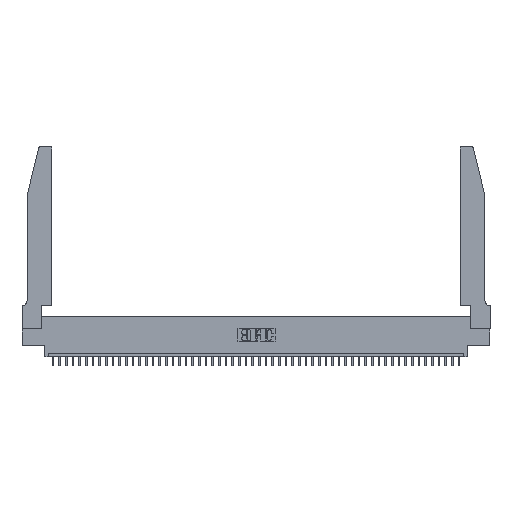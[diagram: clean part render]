
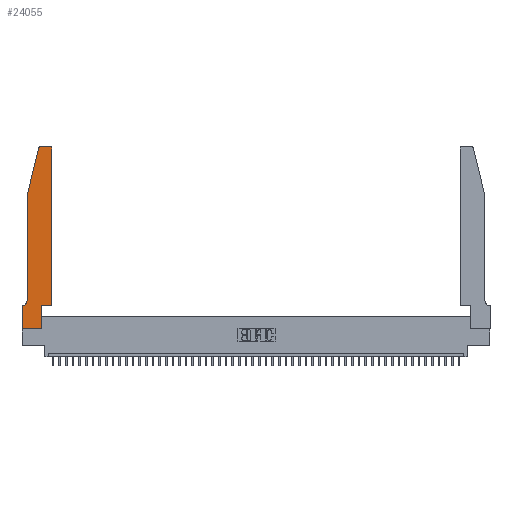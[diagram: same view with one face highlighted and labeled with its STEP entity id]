
A CAD part, top view. The second image highlights one B-rep face of the part: STEP entity #24055.
In plain terms, the highlighted planar face has unit normal (0, 0, 1).
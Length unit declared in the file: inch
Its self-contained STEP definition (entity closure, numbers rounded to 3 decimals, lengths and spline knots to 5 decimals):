
#559 = VECTOR ( 'NONE', #22969, 39.37008 ) ;
#1103 = LINE ( 'NONE', #23574, #22362 ) ;
#1357 = ORIENTED_EDGE ( 'NONE', *, *, #5069, .T. ) ;
#1638 = CARTESIAN_POINT ( 'NONE',  ( 0.0755, 2., 0.37 ) ) ;
#2776 = VERTEX_POINT ( 'NONE', #11115 ) ;
#2872 = DIRECTION ( 'NONE',  ( -1., 0., 0. ) ) ;
#3125 = DIRECTION ( 'NONE',  ( 1., 0., 0. ) ) ;
#4115 = ORIENTED_EDGE ( 'NONE', *, *, #41771, .T. ) ;
#4486 = VECTOR ( 'NONE', #7518, 39.37008 ) ;
#4956 = EDGE_CURVE ( 'NONE', #36904, #31298, #45516, .T. ) ;
#5069 = EDGE_CURVE ( 'NONE', #30565, #15006, #5360, .T. ) ;
#5360 = LINE ( 'NONE', #42380, #559 ) ;
#6706 = DIRECTION ( 'NONE',  ( 1., 0., 0. ) ) ;
#7518 = DIRECTION ( 'NONE',  ( 0., 1., 0. ) ) ;
#7743 = LINE ( 'NONE', #1638, #20049 ) ;
#8378 = CARTESIAN_POINT ( 'NONE',  ( 0.25487, 2.72718, 0.37 ) ) ;
#9094 = LINE ( 'NONE', #27854, #23167 ) ;
#9444 = ORIENTED_EDGE ( 'NONE', *, *, #26801, .T. ) ;
#9681 = AXIS2_PLACEMENT_3D ( 'NONE', #30331, #41600, #33811 ) ;
#9833 = CARTESIAN_POINT ( 'NONE',  ( 0.2865, 0.35, 0.37 ) ) ;
#9986 = ORIENTED_EDGE ( 'NONE', *, *, #24426, .T. ) ;
#10531 = VERTEX_POINT ( 'NONE', #17291 ) ;
#11115 = CARTESIAN_POINT ( 'NONE',  ( 0., 0.35, 0.37 ) ) ;
#11484 = FACE_OUTER_BOUND ( 'NONE', #29767, .T. ) ;
#11718 = CARTESIAN_POINT ( 'NONE',  ( 0.2865, 0., 0.37 ) ) ;
#12061 = DIRECTION ( 'NONE',  ( 0., 1., 0. ) ) ;
#12645 = CARTESIAN_POINT ( 'NONE',  ( 0.0055, 0.35, 0.37 ) ) ;
#12765 = LINE ( 'NONE', #9833, #4486 ) ;
#13331 = CARTESIAN_POINT ( 'NONE',  ( 0.4205, 2.75, 0.37 ) ) ;
#13377 = DIRECTION ( 'NONE',  ( -1., 0., 0. ) ) ;
#14052 = CARTESIAN_POINT ( 'NONE',  ( 0.4205, 2.72, 0.37 ) ) ;
#14626 = AXIS2_PLACEMENT_3D ( 'NONE', #33946, #37298, #3125 ) ;
#15006 = VERTEX_POINT ( 'NONE', #39489 ) ;
#15612 = VECTOR ( 'NONE', #29946, 39.37008 ) ;
#15670 = ORIENTED_EDGE ( 'NONE', *, *, #39494, .T. ) ;
#16817 = AXIS2_PLACEMENT_3D ( 'NONE', #14052, #17802, #6706 ) ;
#17291 = CARTESIAN_POINT ( 'NONE',  ( 0.0755, 0.42, 0.37 ) ) ;
#17571 = EDGE_CURVE ( 'NONE', #15006, #10531, #7743, .T. ) ;
#17802 = DIRECTION ( 'NONE',  ( 0., 0., 1. ) ) ;
#18466 = VERTEX_POINT ( 'NONE', #43878 ) ;
#19421 = VERTEX_POINT ( 'NONE', #13331 ) ;
#20049 = VECTOR ( 'NONE', #35821, 39.37008 ) ;
#20183 = VECTOR ( 'NONE', #25851, 39.37008 ) ;
#20469 = EDGE_CURVE ( 'NONE', #18466, #44618, #1103, .T. ) ;
#21346 = LINE ( 'NONE', #32237, #39133 ) ;
#22362 = VECTOR ( 'NONE', #12061, 39.37008 ) ;
#22926 = VERTEX_POINT ( 'NONE', #47228 ) ;
#22969 = DIRECTION ( 'NONE',  ( -0.239, -0.971, 0. ) ) ;
#23167 = VECTOR ( 'NONE', #41052, 39.37008 ) ;
#23405 = CARTESIAN_POINT ( 'NONE',  ( 0.0055, 0.42, 0.37 ) ) ;
#23574 = CARTESIAN_POINT ( 'NONE',  ( 0.4505, 0.35, 0.37 ) ) ;
#24055 = ADVANCED_FACE ( 'NONE', ( #11484 ), #37603, .T. ) ;
#24426 = EDGE_CURVE ( 'NONE', #2776, #36904, #9094, .T. ) ;
#24615 = CARTESIAN_POINT ( 'NONE',  ( 0.4505, 2.72, 0.37 ) ) ;
#25329 = EDGE_CURVE ( 'NONE', #44618, #19421, #48543, .T. ) ;
#25851 = DIRECTION ( 'NONE',  ( 1., 0., 0. ) ) ;
#26140 = EDGE_CURVE ( 'NONE', #31298, #22926, #12765, .T. ) ;
#26801 = EDGE_CURVE ( 'NONE', #22926, #18466, #30311, .T. ) ;
#27002 = EDGE_CURVE ( 'NONE', #28408, #2776, #21346, .T. ) ;
#27034 = ORIENTED_EDGE ( 'NONE', *, *, #25329, .T. ) ;
#27854 = CARTESIAN_POINT ( 'NONE',  ( 0., 0., 0.37 ) ) ;
#28408 = VERTEX_POINT ( 'NONE', #12645 ) ;
#28414 = ORIENTED_EDGE ( 'NONE', *, *, #26140, .T. ) ;
#28447 = CIRCLE ( 'NONE', #45737, 0.07 ) ;
#29022 = CIRCLE ( 'NONE', #9681, 0.03 ) ;
#29306 = LINE ( 'NONE', #30572, #15612 ) ;
#29571 = ORIENTED_EDGE ( 'NONE', *, *, #41751, .T. ) ;
#29767 = EDGE_LOOP ( 'NONE', ( #15670, #4115, #1357, #40298, #29571, #33514, #9986, #43389, #28414, #9444, #35333, #27034 ) ) ;
#29857 = CARTESIAN_POINT ( 'NONE',  ( 0., 0., 0.37 ) ) ;
#29946 = DIRECTION ( 'NONE',  ( -1., 0., 0. ) ) ;
#30311 = LINE ( 'NONE', #47322, #20183 ) ;
#30331 = CARTESIAN_POINT ( 'NONE',  ( 0.284, 2.72, 0.37 ) ) ;
#30565 = VERTEX_POINT ( 'NONE', #8378 ) ;
#30572 = CARTESIAN_POINT ( 'NONE',  ( 0.2605, 2.75, 0.37 ) ) ;
#31298 = VERTEX_POINT ( 'NONE', #11718 ) ;
#32237 = CARTESIAN_POINT ( 'NONE',  ( 0.0755, 0.35, 0.37 ) ) ;
#33514 = ORIENTED_EDGE ( 'NONE', *, *, #27002, .T. ) ;
#33544 = VERTEX_POINT ( 'NONE', #43995 ) ;
#33746 = DIRECTION ( 'NONE',  ( 0., 0., -1. ) ) ;
#33811 = DIRECTION ( 'NONE',  ( 1., 0., 0. ) ) ;
#33946 = CARTESIAN_POINT ( 'NONE',  ( 0., 0.35, 0.37 ) ) ;
#35333 = ORIENTED_EDGE ( 'NONE', *, *, #20469, .T. ) ;
#35436 = VECTOR ( 'NONE', #37142, 39.37008 ) ;
#35821 = DIRECTION ( 'NONE',  ( 0., -1., 0. ) ) ;
#36904 = VERTEX_POINT ( 'NONE', #47610 ) ;
#37142 = DIRECTION ( 'NONE',  ( 1., 0., 0. ) ) ;
#37298 = DIRECTION ( 'NONE',  ( 0., 0., 1. ) ) ;
#37603 = PLANE ( 'NONE',  #14626 ) ;
#39133 = VECTOR ( 'NONE', #13377, 39.37008 ) ;
#39489 = CARTESIAN_POINT ( 'NONE',  ( 0.0755, 2., 0.37 ) ) ;
#39494 = EDGE_CURVE ( 'NONE', #19421, #33544, #29306, .T. ) ;
#40298 = ORIENTED_EDGE ( 'NONE', *, *, #17571, .T. ) ;
#41052 = DIRECTION ( 'NONE',  ( 0., -1., 0. ) ) ;
#41600 = DIRECTION ( 'NONE',  ( 0., 0., 1. ) ) ;
#41751 = EDGE_CURVE ( 'NONE', #10531, #28408, #28447, .T. ) ;
#41771 = EDGE_CURVE ( 'NONE', #33544, #30565, #29022, .T. ) ;
#42380 = CARTESIAN_POINT ( 'NONE',  ( 0.0755, 2., 0.37 ) ) ;
#43389 = ORIENTED_EDGE ( 'NONE', *, *, #4956, .T. ) ;
#43878 = CARTESIAN_POINT ( 'NONE',  ( 0.4505, 0.35, 0.37 ) ) ;
#43995 = CARTESIAN_POINT ( 'NONE',  ( 0.284, 2.75, 0.37 ) ) ;
#44618 = VERTEX_POINT ( 'NONE', #24615 ) ;
#45516 = LINE ( 'NONE', #29857, #35436 ) ;
#45737 = AXIS2_PLACEMENT_3D ( 'NONE', #23405, #33746, #2872 ) ;
#47228 = CARTESIAN_POINT ( 'NONE',  ( 0.2865, 0.35, 0.37 ) ) ;
#47322 = CARTESIAN_POINT ( 'NONE',  ( 0.4505, 0.35, 0.37 ) ) ;
#47610 = CARTESIAN_POINT ( 'NONE',  ( 0., 0., 0.37 ) ) ;
#48543 = CIRCLE ( 'NONE', #16817, 0.03 ) ;
